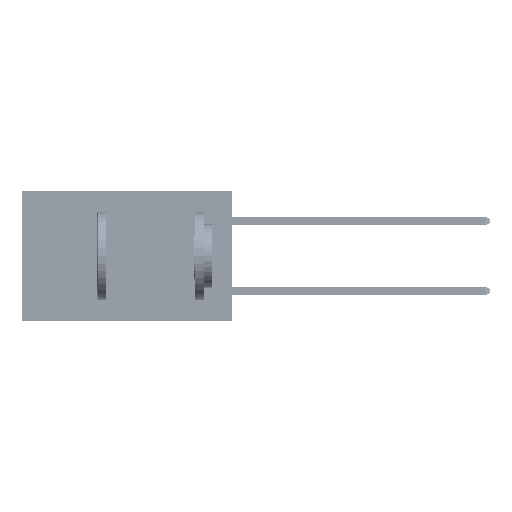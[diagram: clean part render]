
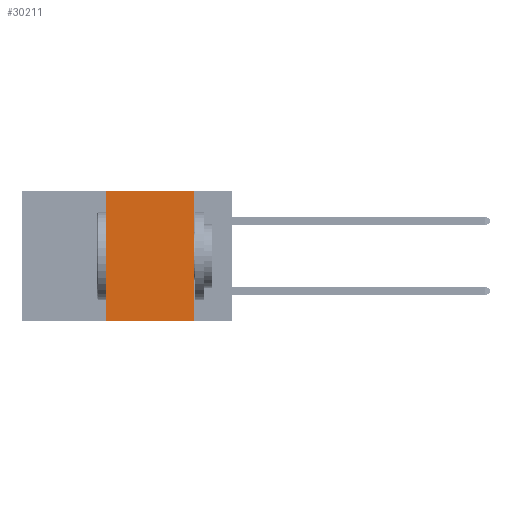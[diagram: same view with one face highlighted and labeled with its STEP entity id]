
A CAD part, left-side view. The second image highlights one B-rep face of the part: STEP entity #30211.
In plain terms, the highlighted planar face has unit normal (-1, 0, 0).
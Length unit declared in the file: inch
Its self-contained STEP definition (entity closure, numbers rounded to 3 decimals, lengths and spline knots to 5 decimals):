
#291 = VECTOR ( 'NONE', #28527, 39.37008 ) ;
#1474 = ORIENTED_EDGE ( 'NONE', *, *, #36453, .F. ) ;
#1930 = VERTEX_POINT ( 'NONE', #31163 ) ;
#2554 = AXIS2_PLACEMENT_3D ( 'NONE', #20389, #32007, #13041 ) ;
#3669 = DIRECTION ( 'NONE',  ( 0., 0., -1. ) ) ;
#4089 = EDGE_CURVE ( 'NONE', #1930, #36566, #21105, .T. ) ;
#5289 = CARTESIAN_POINT ( 'NONE',  ( 0., 0.36, 0. ) ) ;
#6685 = ORIENTED_EDGE ( 'NONE', *, *, #22404, .T. ) ;
#7248 = CARTESIAN_POINT ( 'NONE',  ( 0., 0.11, 0. ) ) ;
#9237 = EDGE_LOOP ( 'NONE', ( #20477, #1474, #17180, #6685 ) ) ;
#10001 = LINE ( 'NONE', #46183, #13056 ) ;
#13041 = DIRECTION ( 'NONE',  ( 0., 0., -1. ) ) ;
#13056 = VECTOR ( 'NONE', #15425, 39.37008 ) ;
#14255 = CARTESIAN_POINT ( 'NONE',  ( 0., 0.6, -0.37 ) ) ;
#15425 = DIRECTION ( 'NONE',  ( 0., -1., 0. ) ) ;
#17180 = ORIENTED_EDGE ( 'NONE', *, *, #4089, .F. ) ;
#17696 = DIRECTION ( 'NONE',  ( 0., -1., 0. ) ) ;
#20389 = CARTESIAN_POINT ( 'NONE',  ( 0., 0.6, 0. ) ) ;
#20477 = ORIENTED_EDGE ( 'NONE', *, *, #46671, .F. ) ;
#21105 = LINE ( 'NONE', #5289, #291 ) ;
#22404 = EDGE_CURVE ( 'NONE', #1930, #38810, #47254, .T. ) ;
#26539 = CARTESIAN_POINT ( 'NONE',  ( 0., 0.11, 0. ) ) ;
#28527 = DIRECTION ( 'NONE',  ( 0., 0., 1. ) ) ;
#29851 = LINE ( 'NONE', #7248, #49442 ) ;
#30211 = ADVANCED_FACE ( 'NONE', ( #41081 ), #32678, .F. ) ;
#31163 = CARTESIAN_POINT ( 'NONE',  ( 0., 0.36, -0.37 ) ) ;
#32007 = DIRECTION ( 'NONE',  ( 1., 0., 0. ) ) ;
#32678 = PLANE ( 'NONE',  #2554 ) ;
#36453 = EDGE_CURVE ( 'NONE', #36566, #37573, #10001, .T. ) ;
#36566 = VERTEX_POINT ( 'NONE', #47040 ) ;
#36862 = VECTOR ( 'NONE', #17696, 39.37008 ) ;
#37573 = VERTEX_POINT ( 'NONE', #26539 ) ;
#38810 = VERTEX_POINT ( 'NONE', #41700 ) ;
#41081 = FACE_OUTER_BOUND ( 'NONE', #9237, .T. ) ;
#41700 = CARTESIAN_POINT ( 'NONE',  ( 0., 0.11, -0.37 ) ) ;
#46183 = CARTESIAN_POINT ( 'NONE',  ( 0., 0.6, 0. ) ) ;
#46671 = EDGE_CURVE ( 'NONE', #37573, #38810, #29851, .T. ) ;
#47040 = CARTESIAN_POINT ( 'NONE',  ( 0., 0.36, 0. ) ) ;
#47254 = LINE ( 'NONE', #14255, #36862 ) ;
#49442 = VECTOR ( 'NONE', #3669, 39.37008 ) ;
